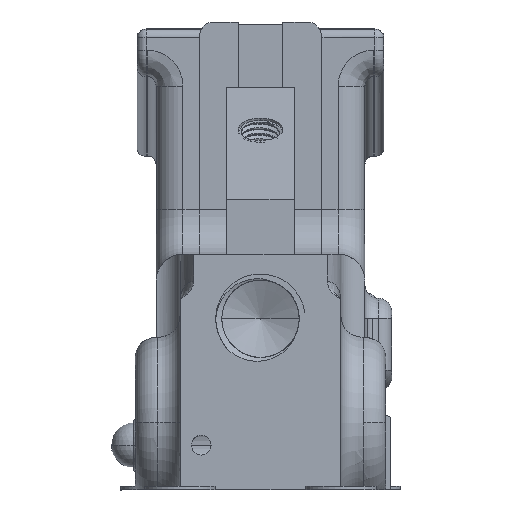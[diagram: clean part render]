
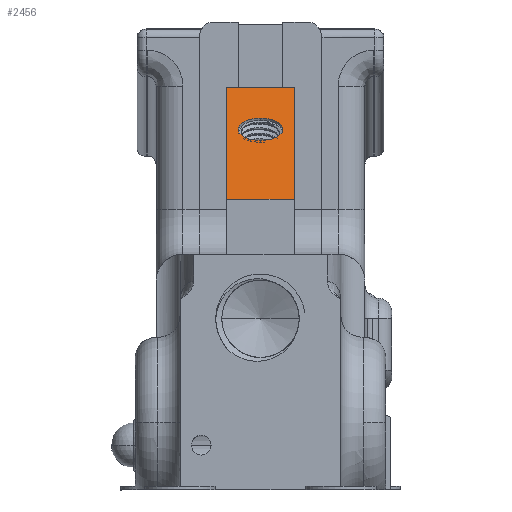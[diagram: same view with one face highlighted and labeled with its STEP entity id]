
A CAD part, left-side view. The second image highlights one B-rep face of the part: STEP entity #2456.
In plain terms, the highlighted planar face has unit normal (-0.5, 0, 0.866).
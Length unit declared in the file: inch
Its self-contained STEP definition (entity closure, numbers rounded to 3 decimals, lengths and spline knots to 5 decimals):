
#820 = LINE ( 'NONE', #84799, #116095 ) ;
#2386 = ORIENTED_EDGE ( 'NONE', *, *, #92960, .T. ) ;
#2456 = ADVANCED_FACE ( 'NONE', ( #96330, #73848 ), #86583, .F. ) ;
#3498 = DIRECTION ( 'NONE',  ( 0., 1., 0. ) ) ;
#3556 = EDGE_CURVE ( 'NONE', #14832, #21380, #48309, .T. ) ;
#7261 = EDGE_CURVE ( 'NONE', #21380, #14832, #72294, .T. ) ;
#10430 = VERTEX_POINT ( 'NONE', #69125 ) ;
#11008 = CARTESIAN_POINT ( 'NONE',  ( -2.7955, 0.46865, 0.34159 ) ) ;
#14335 = ORIENTED_EDGE ( 'NONE', *, *, #3556, .F. ) ;
#14832 = VERTEX_POINT ( 'NONE', #112078 ) ;
#18403 = AXIS2_PLACEMENT_3D ( 'NONE', #113659, #65923, #96039 ) ;
#19271 = DIRECTION ( 'NONE',  ( -0.866, 0., -0.5 ) ) ;
#21380 = VERTEX_POINT ( 'NONE', #67686 ) ;
#22210 = VECTOR ( 'NONE', #115680, 39.37008 ) ;
#22280 = CARTESIAN_POINT ( 'NONE',  ( -1.71633, 0.46865, 0.96465 ) ) ;
#27549 = ORIENTED_EDGE ( 'NONE', *, *, #60084, .T. ) ;
#28029 = CARTESIAN_POINT ( 'NONE',  ( -2.7955, 0.46865, 0.34159 ) ) ;
#32931 = VERTEX_POINT ( 'NONE', #46361 ) ;
#37932 = DIRECTION ( 'NONE',  ( 0.866, 0., 0.5 ) ) ;
#39319 = CARTESIAN_POINT ( 'NONE',  ( -2.7955, 1.53115, 0.34159 ) ) ;
#39479 = LINE ( 'NONE', #39319, #105595 ) ;
#40025 = EDGE_LOOP ( 'NONE', ( #2386, #50270, #51919, #27549 ) ) ;
#41181 = DIRECTION ( 'NONE',  ( 0.866, 0., 0.5 ) ) ;
#46361 = CARTESIAN_POINT ( 'NONE',  ( -1.71633, 1.53115, 0.96465 ) ) ;
#48309 = CIRCLE ( 'NONE', #18403, 0.125 ) ;
#49993 = CARTESIAN_POINT ( 'NONE',  ( -2.11876, 1.34365, 0.7323 ) ) ;
#50270 = ORIENTED_EDGE ( 'NONE', *, *, #118081, .T. ) ;
#51202 = AXIS2_PLACEMENT_3D ( 'NONE', #28029, #85760, #104630 ) ;
#51638 = VERTEX_POINT ( 'NONE', #67969 ) ;
#51919 = ORIENTED_EDGE ( 'NONE', *, *, #101901, .F. ) ;
#54365 = EDGE_LOOP ( 'NONE', ( #14335, #69352 ) ) ;
#60084 = EDGE_CURVE ( 'NONE', #10430, #51638, #820, .T. ) ;
#65923 = DIRECTION ( 'NONE',  ( -0.5, 0., 0.866 ) ) ;
#67686 = CARTESIAN_POINT ( 'NONE',  ( -2.22701, 1.34365, 0.6698 ) ) ;
#67969 = CARTESIAN_POINT ( 'NONE',  ( -1.71633, 1.15615, 0.96465 ) ) ;
#68493 = CARTESIAN_POINT ( 'NONE',  ( -2.7955, 1.53115, 0.34159 ) ) ;
#69125 = CARTESIAN_POINT ( 'NONE',  ( -2.7955, 1.15615, 0.34159 ) ) ;
#69352 = ORIENTED_EDGE ( 'NONE', *, *, #7261, .F. ) ;
#72294 = CIRCLE ( 'NONE', #121967, 0.125 ) ;
#73848 = FACE_BOUND ( 'NONE', #54365, .T. ) ;
#77326 = VERTEX_POINT ( 'NONE', #68493 ) ;
#79258 = LINE ( 'NONE', #22280, #118200 ) ;
#80065 = DIRECTION ( 'NONE',  ( -0.5, 0., 0.866 ) ) ;
#84799 = CARTESIAN_POINT ( 'NONE',  ( -2.7955, 1.15615, 0.34159 ) ) ;
#85760 = DIRECTION ( 'NONE',  ( 0.5, 0., -0.866 ) ) ;
#86583 = PLANE ( 'NONE',  #51202 ) ;
#92960 = EDGE_CURVE ( 'NONE', #51638, #32931, #79258, .T. ) ;
#96039 = DIRECTION ( 'NONE',  ( 0.866, 0., 0.5 ) ) ;
#96330 = FACE_OUTER_BOUND ( 'NONE', #40025, .T. ) ;
#101901 = EDGE_CURVE ( 'NONE', #10430, #77326, #122525, .T. ) ;
#104630 = DIRECTION ( 'NONE',  ( -0.866, 0., -0.5 ) ) ;
#105595 = VECTOR ( 'NONE', #19271, 39.37008 ) ;
#112078 = CARTESIAN_POINT ( 'NONE',  ( -2.01051, 1.34365, 0.7948 ) ) ;
#113659 = CARTESIAN_POINT ( 'NONE',  ( -2.11876, 1.34365, 0.7323 ) ) ;
#115680 = DIRECTION ( 'NONE',  ( 0., 1., 0. ) ) ;
#116095 = VECTOR ( 'NONE', #37932, 39.37008 ) ;
#118081 = EDGE_CURVE ( 'NONE', #32931, #77326, #39479, .T. ) ;
#118200 = VECTOR ( 'NONE', #3498, 39.37008 ) ;
#121967 = AXIS2_PLACEMENT_3D ( 'NONE', #49993, #80065, #41181 ) ;
#122525 = LINE ( 'NONE', #11008, #22210 ) ;
